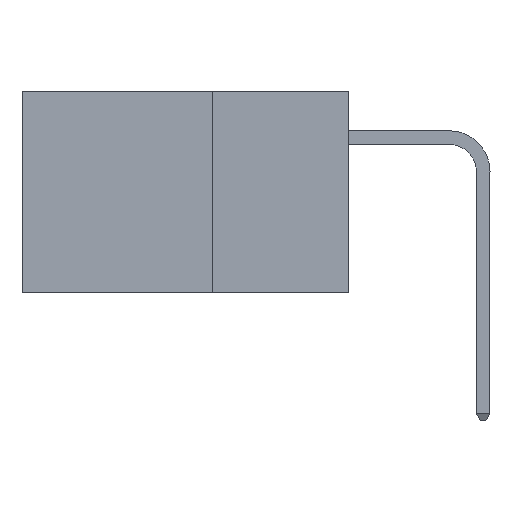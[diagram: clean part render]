
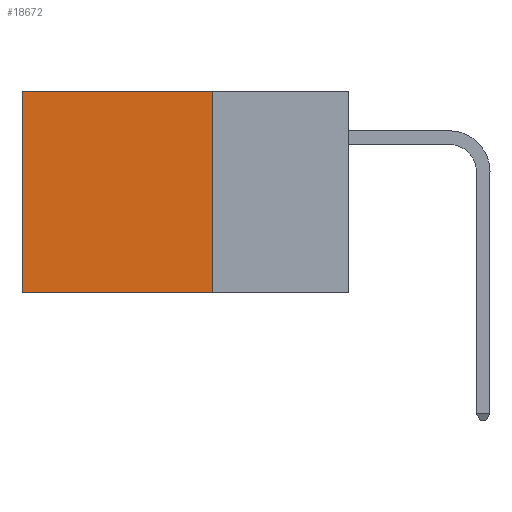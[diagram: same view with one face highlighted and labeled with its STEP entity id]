
A CAD part, left-side view. The second image highlights one B-rep face of the part: STEP entity #18672.
In plain terms, the highlighted planar face has unit normal (-1, 0, 0).
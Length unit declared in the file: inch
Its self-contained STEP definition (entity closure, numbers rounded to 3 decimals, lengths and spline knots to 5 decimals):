
#327 = VERTEX_POINT ( 'NONE', #2806 ) ;
#426 = CARTESIAN_POINT ( 'NONE',  ( 0.2875, 0.25, -0.37 ) ) ;
#1784 = DIRECTION ( 'NONE',  ( 0., 1., 0. ) ) ;
#2806 = CARTESIAN_POINT ( 'NONE',  ( 0.2875, 0.25, 0. ) ) ;
#2940 = CARTESIAN_POINT ( 'NONE',  ( 0.2875, 0.6, 0. ) ) ;
#5079 = LINE ( 'NONE', #2940, #26013 ) ;
#9670 = VECTOR ( 'NONE', #23264, 39.37008 ) ;
#9915 = ORIENTED_EDGE ( 'NONE', *, *, #25968, .F. ) ;
#11471 = LINE ( 'NONE', #426, #9670 ) ;
#13610 = VERTEX_POINT ( 'NONE', #26490 ) ;
#14131 = AXIS2_PLACEMENT_3D ( 'NONE', #34708, #23134, #23252 ) ;
#15215 = EDGE_LOOP ( 'NONE', ( #26985, #9915, #25776, #15695 ) ) ;
#15695 = ORIENTED_EDGE ( 'NONE', *, *, #22940, .T. ) ;
#16150 = LINE ( 'NONE', #21737, #22716 ) ;
#18192 = CARTESIAN_POINT ( 'NONE',  ( 0.2875, 0.6, -0.37 ) ) ;
#18672 = ADVANCED_FACE ( 'NONE', ( #30634 ), #20455, .F. ) ;
#20455 = PLANE ( 'NONE',  #14131 ) ;
#20719 = VERTEX_POINT ( 'NONE', #20869 ) ;
#20869 = CARTESIAN_POINT ( 'NONE',  ( 0.2875, 0.6, 0. ) ) ;
#21737 = CARTESIAN_POINT ( 'NONE',  ( 0.2875, 0.25, 0. ) ) ;
#22354 = DIRECTION ( 'NONE',  ( 0., 0., -1. ) ) ;
#22716 = VECTOR ( 'NONE', #1784, 39.37008 ) ;
#22940 = EDGE_CURVE ( 'NONE', #327, #20719, #16150, .T. ) ;
#23134 = DIRECTION ( 'NONE',  ( 1., 0., 0. ) ) ;
#23252 = DIRECTION ( 'NONE',  ( 0., 0., -1. ) ) ;
#23264 = DIRECTION ( 'NONE',  ( 0., 1., 0. ) ) ;
#25776 = ORIENTED_EDGE ( 'NONE', *, *, #31838, .F. ) ;
#25968 = EDGE_CURVE ( 'NONE', #13610, #32168, #11471, .T. ) ;
#26013 = VECTOR ( 'NONE', #34440, 39.37008 ) ;
#26490 = CARTESIAN_POINT ( 'NONE',  ( 0.2875, 0.25, -0.37 ) ) ;
#26529 = EDGE_CURVE ( 'NONE', #20719, #32168, #5079, .T. ) ;
#26985 = ORIENTED_EDGE ( 'NONE', *, *, #26529, .T. ) ;
#28550 = VECTOR ( 'NONE', #22354, 39.37008 ) ;
#30634 = FACE_OUTER_BOUND ( 'NONE', #15215, .T. ) ;
#31838 = EDGE_CURVE ( 'NONE', #327, #13610, #37057, .T. ) ;
#32168 = VERTEX_POINT ( 'NONE', #18192 ) ;
#33793 = CARTESIAN_POINT ( 'NONE',  ( 0.2875, 0.25, 0. ) ) ;
#34440 = DIRECTION ( 'NONE',  ( 0., 0., -1. ) ) ;
#34708 = CARTESIAN_POINT ( 'NONE',  ( 0.2875, 0.25, 0. ) ) ;
#37057 = LINE ( 'NONE', #33793, #28550 ) ;
